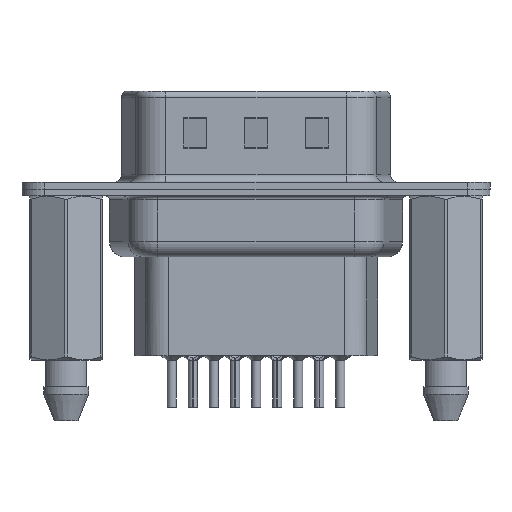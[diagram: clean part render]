
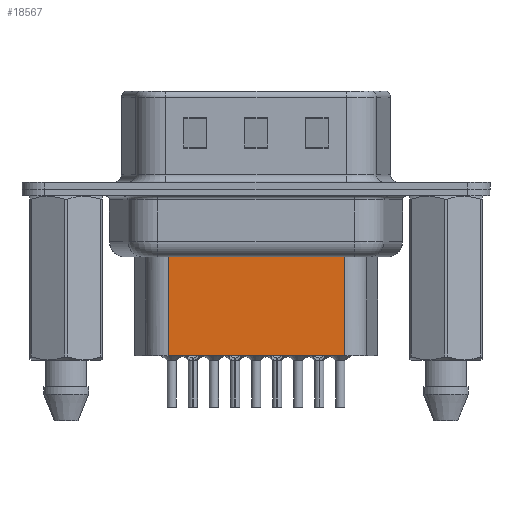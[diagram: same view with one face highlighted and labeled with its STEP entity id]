
A CAD part, front view. The second image highlights one B-rep face of the part: STEP entity #18567.
In plain terms, the highlighted planar face has unit normal (0, -1, 0).
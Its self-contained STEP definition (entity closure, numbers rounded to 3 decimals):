
#1829 = EDGE_CURVE ( 'NONE', #8299, #21624, #10549, .T. ) ;
#2283 = CARTESIAN_POINT ( 'NONE',  ( 6.706, -3.5, -4.097 ) ) ;
#2395 = FACE_OUTER_BOUND ( 'NONE', #15533, .T. ) ;
#2711 = DIRECTION ( 'NONE',  ( -1., 0., 0. ) ) ;
#3202 = VERTEX_POINT ( 'NONE', #11304 ) ;
#3250 = AXIS2_PLACEMENT_3D ( 'NONE', #19238, #7168, #9296 ) ;
#3974 = CARTESIAN_POINT ( 'NONE',  ( 6.706, -3.5, -10.95 ) ) ;
#4418 = LINE ( 'NONE', #7930, #18296 ) ;
#6058 = VERTEX_POINT ( 'NONE', #2283 ) ;
#6880 = EDGE_CURVE ( 'NONE', #3202, #8299, #14197, .T. ) ;
#7168 = DIRECTION ( 'NONE',  ( 0., -1., 0. ) ) ;
#7930 = CARTESIAN_POINT ( 'NONE',  ( 6.459, -3.5, -4.097 ) ) ;
#8299 = VERTEX_POINT ( 'NONE', #15502 ) ;
#8381 = ORIENTED_EDGE ( 'NONE', *, *, #13883, .T. ) ;
#8803 = CARTESIAN_POINT ( 'NONE',  ( 6.706, -3.5, -10.95 ) ) ;
#8967 = PLANE ( 'NONE',  #3250 ) ;
#9296 = DIRECTION ( 'NONE',  ( 1., 0., 0. ) ) ;
#9462 = ORIENTED_EDGE ( 'NONE', *, *, #6880, .F. ) ;
#10549 = LINE ( 'NONE', #3974, #12381 ) ;
#11304 = CARTESIAN_POINT ( 'NONE',  ( 18.294, -3.5, -4.097 ) ) ;
#12381 = VECTOR ( 'NONE', #21043, 1000. ) ;
#12418 = EDGE_CURVE ( 'NONE', #6058, #21624, #21063, .T. ) ;
#13883 = EDGE_CURVE ( 'NONE', #3202, #6058, #4418, .T. ) ;
#14197 = LINE ( 'NONE', #19373, #20234 ) ;
#14501 = CARTESIAN_POINT ( 'NONE',  ( 6.706, -3.5, -3.1 ) ) ;
#15502 = CARTESIAN_POINT ( 'NONE',  ( 18.294, -3.5, -10.95 ) ) ;
#15533 = EDGE_LOOP ( 'NONE', ( #9462, #8381, #18716, #18459 ) ) ;
#16984 = VECTOR ( 'NONE', #21275, 1000. ) ;
#17468 = DIRECTION ( 'NONE',  ( 0., 0., -1. ) ) ;
#18296 = VECTOR ( 'NONE', #2711, 1000. ) ;
#18459 = ORIENTED_EDGE ( 'NONE', *, *, #1829, .F. ) ;
#18567 = ADVANCED_FACE ( 'NONE', ( #2395 ), #8967, .T. ) ;
#18716 = ORIENTED_EDGE ( 'NONE', *, *, #12418, .T. ) ;
#19238 = CARTESIAN_POINT ( 'NONE',  ( 6.706, -3.5, -3.1 ) ) ;
#19373 = CARTESIAN_POINT ( 'NONE',  ( 18.294, -3.5, -3.1 ) ) ;
#20234 = VECTOR ( 'NONE', #17468, 1000. ) ;
#21043 = DIRECTION ( 'NONE',  ( -1., 0., 0. ) ) ;
#21063 = LINE ( 'NONE', #14501, #16984 ) ;
#21275 = DIRECTION ( 'NONE',  ( 0., 0., -1. ) ) ;
#21624 = VERTEX_POINT ( 'NONE', #8803 ) ;
